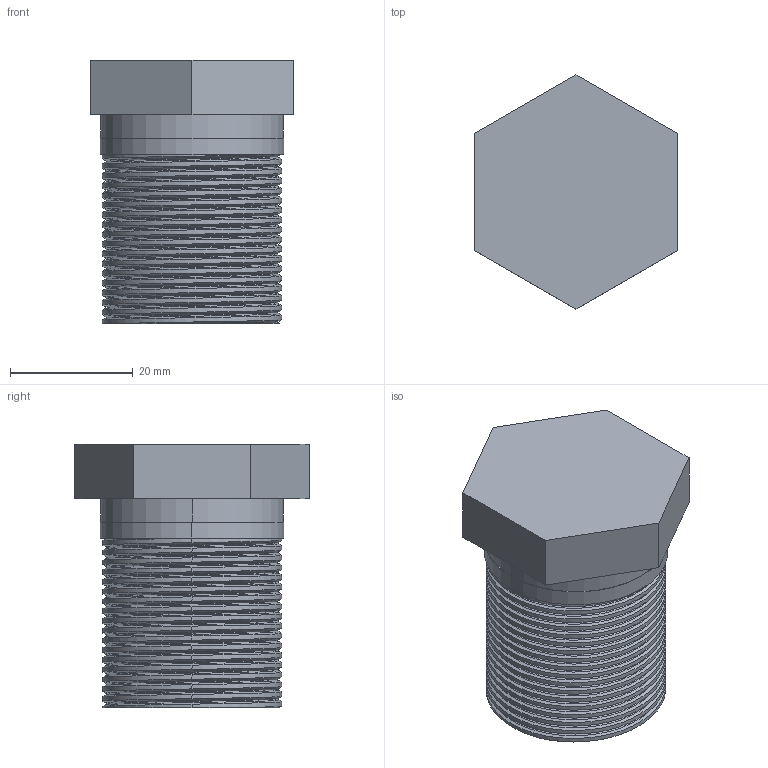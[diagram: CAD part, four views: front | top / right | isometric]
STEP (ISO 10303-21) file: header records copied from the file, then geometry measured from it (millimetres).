
FILE_DESCRIPTION(('FreeCAD Model'),'2;1');
FILE_NAME('buffer retainer bolt.step' ,'2015-07-10T13:11:47',('Author'),(''), 'Open CASCADE STEP processor 6.8','FreeCAD','Unknown');
FILE_SCHEMA(('AUTOMOTIVE_DESIGN_CC2 { 1 2 10303 214 -1 1 5 4 }'));
Products named in the file (1): Pocket
Bounding box: 33 x 38.1 x 42.94 mm (x, y, z)
Volume: 15468.6 mm3; surface area: 10069.2 mm2
Topology: 1 solids, 1 shells, 181 faces, 521 edges, 344 vertices
Faces by surface type: cylinder 83, plane 53, bspline 40, cone 5
Entity records: 53449 total; most frequent: CARTESIAN_POINT 45669, B_SPLINE_CURVE_WITH_KNOTS 1303, ORIENTED_EDGE 1042, PCURVE 1042, DEFINITIONAL_REPRESENTATION 1042, DIRECTION 566, EDGE_CURVE 521, SURFACE_CURVE 521
